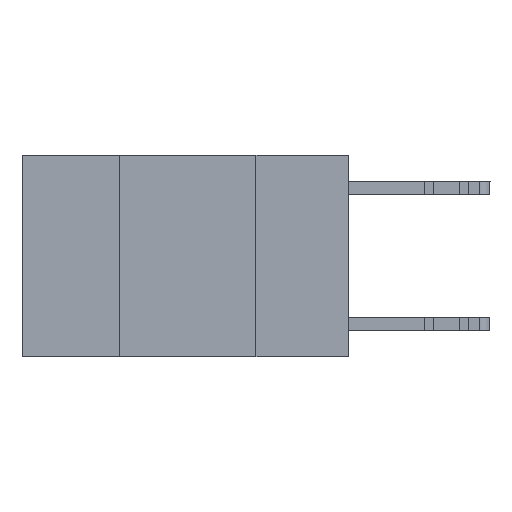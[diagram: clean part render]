
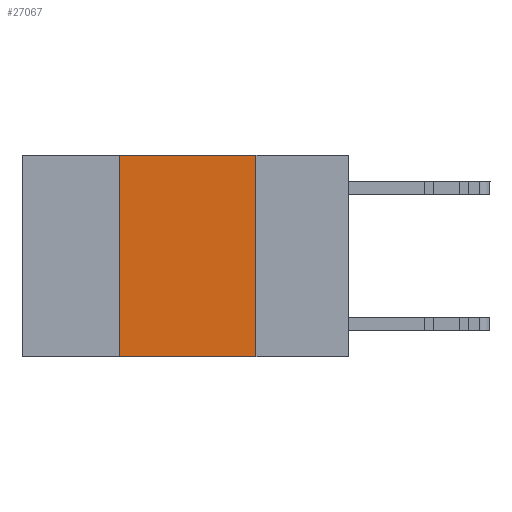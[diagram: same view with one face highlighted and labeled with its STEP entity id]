
A CAD part, left-side view. The second image highlights one B-rep face of the part: STEP entity #27067.
In plain terms, the highlighted planar face has unit normal (-1, 0, 0).
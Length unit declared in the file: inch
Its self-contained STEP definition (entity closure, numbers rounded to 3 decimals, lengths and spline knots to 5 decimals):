
#474 = CARTESIAN_POINT ( 'NONE',  ( 0., 0.6, 0. ) ) ;
#796 = ORIENTED_EDGE ( 'NONE', *, *, #19714, .F. ) ;
#1439 = VECTOR ( 'NONE', #15972, 39.37008 ) ;
#1515 = VECTOR ( 'NONE', #20267, 39.37008 ) ;
#5019 = DIRECTION ( 'NONE',  ( 0., 0., -1. ) ) ;
#5430 = EDGE_LOOP ( 'NONE', ( #18514, #796, #20716, #29292 ) ) ;
#7573 = VECTOR ( 'NONE', #24390, 39.37008 ) ;
#8878 = CARTESIAN_POINT ( 'NONE',  ( 0., 0.6, 0. ) ) ;
#9593 = CARTESIAN_POINT ( 'NONE',  ( 0., 0.42, 0. ) ) ;
#10348 = FACE_OUTER_BOUND ( 'NONE', #5430, .T. ) ;
#10540 = CARTESIAN_POINT ( 'NONE',  ( 0., 0.42, 0. ) ) ;
#10998 = DIRECTION ( 'NONE',  ( 0., -1., 0. ) ) ;
#12065 = CARTESIAN_POINT ( 'NONE',  ( 0., 0.42, -0.37 ) ) ;
#12881 = PLANE ( 'NONE',  #13153 ) ;
#13018 = VERTEX_POINT ( 'NONE', #9593 ) ;
#13153 = AXIS2_PLACEMENT_3D ( 'NONE', #474, #28925, #5019 ) ;
#13377 = CARTESIAN_POINT ( 'NONE',  ( 0., 0.6, -0.37 ) ) ;
#15750 = VERTEX_POINT ( 'NONE', #17780 ) ;
#15972 = DIRECTION ( 'NONE',  ( 0., -1., 0. ) ) ;
#16577 = VECTOR ( 'NONE', #10998, 39.37008 ) ;
#17780 = CARTESIAN_POINT ( 'NONE',  ( 0., 0.17, 0. ) ) ;
#17931 = LINE ( 'NONE', #13377, #16577 ) ;
#18080 = LINE ( 'NONE', #25304, #1515 ) ;
#18085 = CARTESIAN_POINT ( 'NONE',  ( 0., 0.17, -0.37 ) ) ;
#18514 = ORIENTED_EDGE ( 'NONE', *, *, #24925, .F. ) ;
#18621 = LINE ( 'NONE', #8878, #1439 ) ;
#19413 = VERTEX_POINT ( 'NONE', #12065 ) ;
#19714 = EDGE_CURVE ( 'NONE', #13018, #15750, #18621, .T. ) ;
#20267 = DIRECTION ( 'NONE',  ( 0., 0., -1. ) ) ;
#20716 = ORIENTED_EDGE ( 'NONE', *, *, #26066, .F. ) ;
#24390 = DIRECTION ( 'NONE',  ( 0., 0., 1. ) ) ;
#24925 = EDGE_CURVE ( 'NONE', #15750, #26182, #18080, .T. ) ;
#24927 = EDGE_CURVE ( 'NONE', #19413, #26182, #17931, .T. ) ;
#25304 = CARTESIAN_POINT ( 'NONE',  ( 0., 0.17, 0. ) ) ;
#26066 = EDGE_CURVE ( 'NONE', #19413, #13018, #27374, .T. ) ;
#26182 = VERTEX_POINT ( 'NONE', #18085 ) ;
#27067 = ADVANCED_FACE ( 'NONE', ( #10348 ), #12881, .F. ) ;
#27374 = LINE ( 'NONE', #10540, #7573 ) ;
#28925 = DIRECTION ( 'NONE',  ( 1., 0., 0. ) ) ;
#29292 = ORIENTED_EDGE ( 'NONE', *, *, #24927, .T. ) ;
